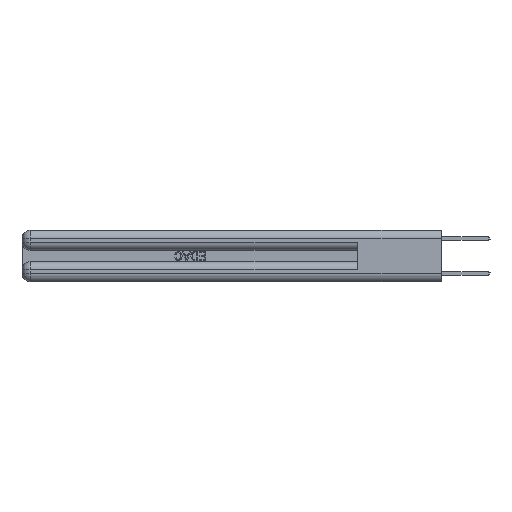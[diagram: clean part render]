
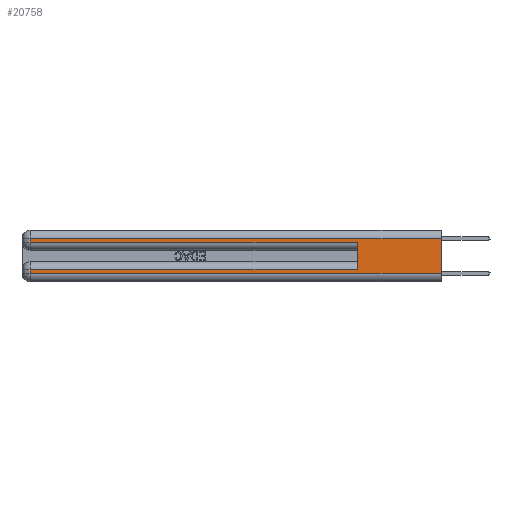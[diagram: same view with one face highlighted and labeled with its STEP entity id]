
A CAD part, left-side view. The second image highlights one B-rep face of the part: STEP entity #20758.
In plain terms, the highlighted planar face has unit normal (-1, 0, 0).
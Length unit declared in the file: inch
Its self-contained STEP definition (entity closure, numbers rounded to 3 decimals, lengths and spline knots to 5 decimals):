
#263 = ORIENTED_EDGE ( 'NONE', *, *, #12486, .T. ) ;
#1834 = CARTESIAN_POINT ( 'NONE',  ( 0., 0.6, 0.085 ) ) ;
#1885 = VERTEX_POINT ( 'NONE', #6538 ) ;
#2305 = CARTESIAN_POINT ( 'NONE',  ( 0., 0., 0.37 ) ) ;
#2464 = DIRECTION ( 'NONE',  ( 0., 0., -1. ) ) ;
#3379 = VECTOR ( 'NONE', #29399, 39.37008 ) ;
#3598 = CARTESIAN_POINT ( 'NONE',  ( 0., 0., 0.31 ) ) ;
#3776 = VERTEX_POINT ( 'NONE', #30200 ) ;
#6538 = CARTESIAN_POINT ( 'NONE',  ( 0., 2.94, 0.285 ) ) ;
#7607 = EDGE_CURVE ( 'NONE', #31489, #31678, #19769, .T. ) ;
#8231 = LINE ( 'NONE', #18272, #9642 ) ;
#8332 = ORIENTED_EDGE ( 'NONE', *, *, #9389, .T. ) ;
#8445 = VECTOR ( 'NONE', #9085, 39.37008 ) ;
#9085 = DIRECTION ( 'NONE',  ( 0., 1., 0. ) ) ;
#9132 = VERTEX_POINT ( 'NONE', #15020 ) ;
#9389 = EDGE_CURVE ( 'NONE', #1885, #16293, #21244, .T. ) ;
#9642 = VECTOR ( 'NONE', #15493, 39.37008 ) ;
#9662 = EDGE_CURVE ( 'NONE', #26635, #9132, #10359, .T. ) ;
#10058 = DIRECTION ( 'NONE',  ( 1., 0., 0. ) ) ;
#10359 = LINE ( 'NONE', #30445, #11153 ) ;
#10551 = FACE_OUTER_BOUND ( 'NONE', #25373, .T. ) ;
#11153 = VECTOR ( 'NONE', #21044, 39.37008 ) ;
#11715 = EDGE_CURVE ( 'NONE', #31489, #16293, #28877, .T. ) ;
#11851 = CARTESIAN_POINT ( 'NONE',  ( 0., 2.94, 0.37 ) ) ;
#11943 = LINE ( 'NONE', #13769, #3379 ) ;
#11974 = ORIENTED_EDGE ( 'NONE', *, *, #26647, .F. ) ;
#12148 = ORIENTED_EDGE ( 'NONE', *, *, #25123, .T. ) ;
#12486 = EDGE_CURVE ( 'NONE', #9132, #1885, #18866, .T. ) ;
#12726 = VECTOR ( 'NONE', #21882, 39.37008 ) ;
#13018 = EDGE_CURVE ( 'NONE', #3776, #31440, #11943, .T. ) ;
#13255 = VECTOR ( 'NONE', #26518, 39.37008 ) ;
#13769 = CARTESIAN_POINT ( 'NONE',  ( 0., 0., 0.06 ) ) ;
#15020 = CARTESIAN_POINT ( 'NONE',  ( 0., 2.94, 0.31 ) ) ;
#15142 = LINE ( 'NONE', #11851, #12726 ) ;
#15493 = DIRECTION ( 'NONE',  ( 0., 0., -1. ) ) ;
#16245 = DIRECTION ( 'NONE',  ( 0., 0., -1. ) ) ;
#16293 = VERTEX_POINT ( 'NONE', #22925 ) ;
#16466 = CARTESIAN_POINT ( 'NONE',  ( 0., 0., 0.285 ) ) ;
#18272 = CARTESIAN_POINT ( 'NONE',  ( 0., 0., 0.37 ) ) ;
#18764 = CARTESIAN_POINT ( 'NONE',  ( 0., 2.94, 0.085 ) ) ;
#18823 = DIRECTION ( 'NONE',  ( 0., 0., 1. ) ) ;
#18866 = LINE ( 'NONE', #23659, #32304 ) ;
#19769 = LINE ( 'NONE', #24402, #8445 ) ;
#19853 = ORIENTED_EDGE ( 'NONE', *, *, #9662, .T. ) ;
#20401 = ORIENTED_EDGE ( 'NONE', *, *, #13018, .T. ) ;
#20758 = ADVANCED_FACE ( 'NONE', ( #10551 ), #27508, .F. ) ;
#20810 = CARTESIAN_POINT ( 'NONE',  ( 0., 0.6, 0.145 ) ) ;
#21044 = DIRECTION ( 'NONE',  ( 0., 1., 0. ) ) ;
#21244 = LINE ( 'NONE', #16466, #13255 ) ;
#21882 = DIRECTION ( 'NONE',  ( 0., 0., -1. ) ) ;
#22017 = ORIENTED_EDGE ( 'NONE', *, *, #11715, .F. ) ;
#22073 = AXIS2_PLACEMENT_3D ( 'NONE', #2305, #10058, #2464 ) ;
#22415 = CARTESIAN_POINT ( 'NONE',  ( 0., 0., 0.06 ) ) ;
#22925 = CARTESIAN_POINT ( 'NONE',  ( 0., 0.6, 0.285 ) ) ;
#23659 = CARTESIAN_POINT ( 'NONE',  ( 0., 2.94, 0.37 ) ) ;
#23870 = VECTOR ( 'NONE', #18823, 39.37008 ) ;
#24390 = ORIENTED_EDGE ( 'NONE', *, *, #7607, .T. ) ;
#24402 = CARTESIAN_POINT ( 'NONE',  ( 0., 0., 0.085 ) ) ;
#25123 = EDGE_CURVE ( 'NONE', #31678, #3776, #15142, .T. ) ;
#25373 = EDGE_LOOP ( 'NONE', ( #11974, #19853, #263, #8332, #22017, #24390, #12148, #20401 ) ) ;
#26518 = DIRECTION ( 'NONE',  ( 0., -1., 0. ) ) ;
#26635 = VERTEX_POINT ( 'NONE', #3598 ) ;
#26647 = EDGE_CURVE ( 'NONE', #26635, #31440, #8231, .T. ) ;
#27508 = PLANE ( 'NONE',  #22073 ) ;
#28877 = LINE ( 'NONE', #20810, #23870 ) ;
#29399 = DIRECTION ( 'NONE',  ( 0., -1., 0. ) ) ;
#30200 = CARTESIAN_POINT ( 'NONE',  ( 0., 2.94, 0.06 ) ) ;
#30445 = CARTESIAN_POINT ( 'NONE',  ( 0., 0., 0.31 ) ) ;
#31440 = VERTEX_POINT ( 'NONE', #22415 ) ;
#31489 = VERTEX_POINT ( 'NONE', #1834 ) ;
#31678 = VERTEX_POINT ( 'NONE', #18764 ) ;
#32304 = VECTOR ( 'NONE', #16245, 39.37008 ) ;
